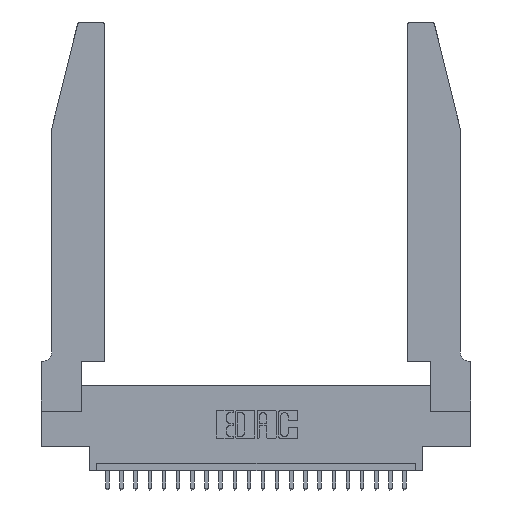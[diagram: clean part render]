
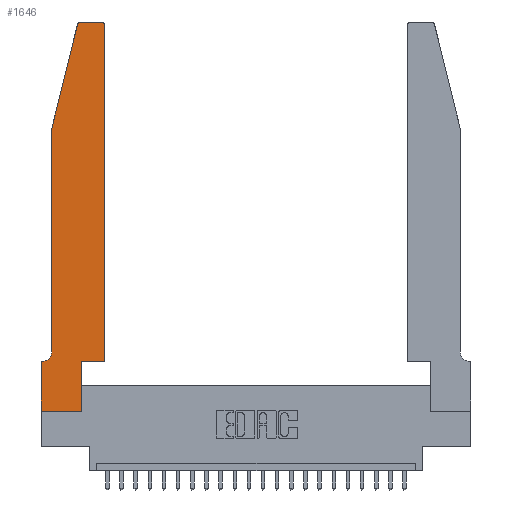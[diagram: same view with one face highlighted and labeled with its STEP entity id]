
A CAD part, top view. The second image highlights one B-rep face of the part: STEP entity #1646.
In plain terms, the highlighted planar face has unit normal (0, 0, 1).
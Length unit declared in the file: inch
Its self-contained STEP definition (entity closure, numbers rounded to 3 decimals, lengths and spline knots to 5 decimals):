
#55 = FACE_OUTER_BOUND ( 'NONE', #18431, .T. ) ;
#68 = DIRECTION ( 'NONE',  ( 1., 0., 0. ) ) ;
#208 = CARTESIAN_POINT ( 'NONE',  ( 0.284, 2.75, 0.37 ) ) ;
#312 = EDGE_CURVE ( 'NONE', #6180, #19518, #15255, .T. ) ;
#532 = CIRCLE ( 'NONE', #7375, 0.03 ) ;
#584 = VERTEX_POINT ( 'NONE', #1155 ) ;
#723 = CARTESIAN_POINT ( 'NONE',  ( 0.0755, 0.42, 0.37 ) ) ;
#728 = CIRCLE ( 'NONE', #8750, 0.07 ) ;
#1155 = CARTESIAN_POINT ( 'NONE',  ( 0.4205, 2.75, 0.37 ) ) ;
#1363 = EDGE_CURVE ( 'NONE', #21183, #6180, #16993, .T. ) ;
#1646 = ADVANCED_FACE ( 'NONE', ( #55 ), #16715, .T. ) ;
#2006 = CARTESIAN_POINT ( 'NONE',  ( 0.4505, 2.72, 0.37 ) ) ;
#2053 = EDGE_CURVE ( 'NONE', #11092, #6720, #10812, .T. ) ;
#2136 = EDGE_CURVE ( 'NONE', #6720, #6300, #16658, .T. ) ;
#2551 = VECTOR ( 'NONE', #10358, 39.37008 ) ;
#2966 = LINE ( 'NONE', #11629, #3794 ) ;
#3114 = DIRECTION ( 'NONE',  ( -1., 0., 0. ) ) ;
#3687 = EDGE_CURVE ( 'NONE', #8812, #11092, #532, .T. ) ;
#3794 = VECTOR ( 'NONE', #17111, 39.37008 ) ;
#4140 = EDGE_CURVE ( 'NONE', #13958, #14805, #8370, .T. ) ;
#4387 = ORIENTED_EDGE ( 'NONE', *, *, #13784, .T. ) ;
#4451 = LINE ( 'NONE', #20466, #11759 ) ;
#4954 = CARTESIAN_POINT ( 'NONE',  ( 0.0755, 2., 0.37 ) ) ;
#5697 = DIRECTION ( 'NONE',  ( 0., 0., 1. ) ) ;
#6180 = VERTEX_POINT ( 'NONE', #9956 ) ;
#6204 = EDGE_CURVE ( 'NONE', #14550, #584, #22881, .T. ) ;
#6300 = VERTEX_POINT ( 'NONE', #723 ) ;
#6720 = VERTEX_POINT ( 'NONE', #4954 ) ;
#6722 = CARTESIAN_POINT ( 'NONE',  ( 0.0755, 2., 0.37 ) ) ;
#7375 = AXIS2_PLACEMENT_3D ( 'NONE', #11233, #22268, #68 ) ;
#8370 = LINE ( 'NONE', #12165, #2551 ) ;
#8750 = AXIS2_PLACEMENT_3D ( 'NONE', #9193, #22270, #12953 ) ;
#8812 = VERTEX_POINT ( 'NONE', #208 ) ;
#9141 = ORIENTED_EDGE ( 'NONE', *, *, #4140, .T. ) ;
#9193 = CARTESIAN_POINT ( 'NONE',  ( 0.0055, 0.42, 0.37 ) ) ;
#9483 = CARTESIAN_POINT ( 'NONE',  ( 0.2865, 0., 0.37 ) ) ;
#9500 = LINE ( 'NONE', #19830, #11854 ) ;
#9672 = CARTESIAN_POINT ( 'NONE',  ( 0., 0., 0.37 ) ) ;
#9851 = ORIENTED_EDGE ( 'NONE', *, *, #14756, .T. ) ;
#9956 = CARTESIAN_POINT ( 'NONE',  ( 0.2865, 0.35, 0.37 ) ) ;
#10351 = DIRECTION ( 'NONE',  ( 1., 0., 0. ) ) ;
#10358 = DIRECTION ( 'NONE',  ( -1., 0., 0. ) ) ;
#10812 = LINE ( 'NONE', #6722, #12266 ) ;
#10874 = DIRECTION ( 'NONE',  ( 0., 1., 0. ) ) ;
#11092 = VERTEX_POINT ( 'NONE', #20442 ) ;
#11233 = CARTESIAN_POINT ( 'NONE',  ( 0.284, 2.72, 0.37 ) ) ;
#11382 = ORIENTED_EDGE ( 'NONE', *, *, #1363, .T. ) ;
#11483 = ORIENTED_EDGE ( 'NONE', *, *, #20932, .T. ) ;
#11629 = CARTESIAN_POINT ( 'NONE',  ( 0.4505, 0.35, 0.37 ) ) ;
#11676 = CARTESIAN_POINT ( 'NONE',  ( 0.0055, 0.35, 0.37 ) ) ;
#11759 = VECTOR ( 'NONE', #22290, 39.37008 ) ;
#11854 = VECTOR ( 'NONE', #23361, 39.37008 ) ;
#12165 = CARTESIAN_POINT ( 'NONE',  ( 0.0755, 0.35, 0.37 ) ) ;
#12266 = VECTOR ( 'NONE', #21130, 39.37008 ) ;
#12329 = EDGE_CURVE ( 'NONE', #6300, #13958, #728, .T. ) ;
#12852 = VECTOR ( 'NONE', #23390, 39.37008 ) ;
#12953 = DIRECTION ( 'NONE',  ( -1., 0., 0. ) ) ;
#13633 = ORIENTED_EDGE ( 'NONE', *, *, #3687, .T. ) ;
#13784 = EDGE_CURVE ( 'NONE', #23417, #21183, #4451, .T. ) ;
#13802 = CARTESIAN_POINT ( 'NONE',  ( 0.2605, 2.75, 0.37 ) ) ;
#13958 = VERTEX_POINT ( 'NONE', #11676 ) ;
#14131 = DIRECTION ( 'NONE',  ( 1., 0., 0. ) ) ;
#14547 = CARTESIAN_POINT ( 'NONE',  ( 0.2865, 0.35, 0.37 ) ) ;
#14550 = VERTEX_POINT ( 'NONE', #2006 ) ;
#14694 = AXIS2_PLACEMENT_3D ( 'NONE', #20348, #5697, #20427 ) ;
#14756 = EDGE_CURVE ( 'NONE', #19518, #14550, #2966, .T. ) ;
#14805 = VERTEX_POINT ( 'NONE', #22944 ) ;
#14845 = VECTOR ( 'NONE', #3114, 39.37008 ) ;
#15247 = AXIS2_PLACEMENT_3D ( 'NONE', #16241, #16084, #14131 ) ;
#15255 = LINE ( 'NONE', #20649, #17597 ) ;
#15832 = ORIENTED_EDGE ( 'NONE', *, *, #6204, .T. ) ;
#16084 = DIRECTION ( 'NONE',  ( 0., 0., 1. ) ) ;
#16241 = CARTESIAN_POINT ( 'NONE',  ( 0.4205, 2.72, 0.37 ) ) ;
#16298 = LINE ( 'NONE', #13802, #14845 ) ;
#16658 = LINE ( 'NONE', #19702, #12852 ) ;
#16715 = PLANE ( 'NONE',  #14694 ) ;
#16913 = EDGE_CURVE ( 'NONE', #584, #8812, #16298, .T. ) ;
#16993 = LINE ( 'NONE', #14547, #19313 ) ;
#17111 = DIRECTION ( 'NONE',  ( 0., 1., 0. ) ) ;
#17470 = ORIENTED_EDGE ( 'NONE', *, *, #16913, .T. ) ;
#17597 = VECTOR ( 'NONE', #10351, 39.37008 ) ;
#17626 = ORIENTED_EDGE ( 'NONE', *, *, #2053, .T. ) ;
#17988 = ORIENTED_EDGE ( 'NONE', *, *, #312, .T. ) ;
#18431 = EDGE_LOOP ( 'NONE', ( #17470, #13633, #17626, #18456, #19944, #9141, #11483, #4387, #11382, #17988, #9851, #15832 ) ) ;
#18456 = ORIENTED_EDGE ( 'NONE', *, *, #2136, .T. ) ;
#19313 = VECTOR ( 'NONE', #10874, 39.37008 ) ;
#19518 = VERTEX_POINT ( 'NONE', #22091 ) ;
#19702 = CARTESIAN_POINT ( 'NONE',  ( 0.0755, 2., 0.37 ) ) ;
#19830 = CARTESIAN_POINT ( 'NONE',  ( 0., 0., 0.37 ) ) ;
#19944 = ORIENTED_EDGE ( 'NONE', *, *, #12329, .T. ) ;
#20348 = CARTESIAN_POINT ( 'NONE',  ( 0., 0.35, 0.37 ) ) ;
#20427 = DIRECTION ( 'NONE',  ( 1., 0., 0. ) ) ;
#20442 = CARTESIAN_POINT ( 'NONE',  ( 0.25487, 2.72718, 0.37 ) ) ;
#20466 = CARTESIAN_POINT ( 'NONE',  ( 0., 0., 0.37 ) ) ;
#20649 = CARTESIAN_POINT ( 'NONE',  ( 0.4505, 0.35, 0.37 ) ) ;
#20932 = EDGE_CURVE ( 'NONE', #14805, #23417, #9500, .T. ) ;
#21130 = DIRECTION ( 'NONE',  ( -0.239, -0.971, 0. ) ) ;
#21183 = VERTEX_POINT ( 'NONE', #9483 ) ;
#22091 = CARTESIAN_POINT ( 'NONE',  ( 0.4505, 0.35, 0.37 ) ) ;
#22268 = DIRECTION ( 'NONE',  ( 0., 0., 1. ) ) ;
#22270 = DIRECTION ( 'NONE',  ( 0., 0., -1. ) ) ;
#22290 = DIRECTION ( 'NONE',  ( 1., 0., 0. ) ) ;
#22881 = CIRCLE ( 'NONE', #15247, 0.03 ) ;
#22944 = CARTESIAN_POINT ( 'NONE',  ( 0., 0.35, 0.37 ) ) ;
#23361 = DIRECTION ( 'NONE',  ( 0., -1., 0. ) ) ;
#23390 = DIRECTION ( 'NONE',  ( 0., -1., 0. ) ) ;
#23417 = VERTEX_POINT ( 'NONE', #9672 ) ;
